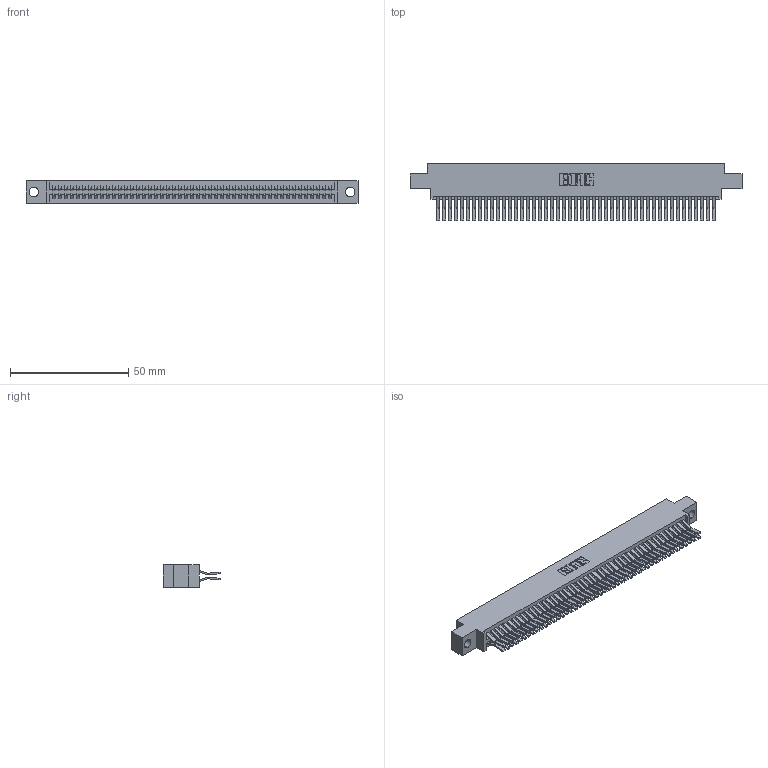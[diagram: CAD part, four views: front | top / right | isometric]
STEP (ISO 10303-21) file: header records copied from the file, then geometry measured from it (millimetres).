
FILE_DESCRIPTION (( 'STEP AP203' ), '1' );
FILE_NAME ('345-094-560-804.STEP', '2018-10-05T02:58:15', ( '' ), ( '' ), 'SwSTEP 2.0', 'SolidWorks 2016', '' );
FILE_SCHEMA (( 'CONFIG_CONTROL_DESIGN' ));
Length unit declared in the file: inch
Products named in the file (3): 345-094-560-804; 345-292-001_560 Tail; 345 Part_0.170 Offset - 0.156 Dia-TH
Assembly tree (95 placements, depth 2):
  345-094-560-804
    345 Part_0.170 Offset - 0.156 Dia-TH
    345-292-001_560 Tail  x94
Bounding box: 140.59 x 24.45 x 9.4 mm (x, y, z)
Volume: 14118.3 mm3; surface area: 22509.3 mm2
Topology: 95 solids, 95 shells, 5018 faces, 14923 edges, 9822 vertices
Faces by surface type: plane 3186, cylinder 1832
Entity records: 36427 total; most frequent: CARTESIAN_POINT 6104, ORIENTED_EDGE 6038, DIRECTION 5379, EDGE_CURVE 3019, VECTOR 2695, LINE 2695, VERTEX_POINT 2010, AXIS2_PLACEMENT_3D 1342
